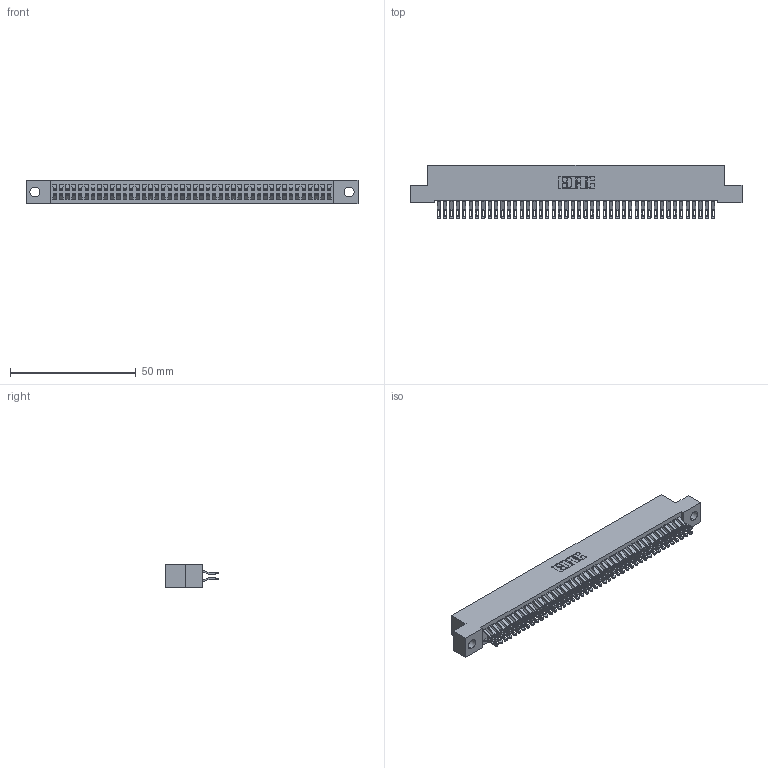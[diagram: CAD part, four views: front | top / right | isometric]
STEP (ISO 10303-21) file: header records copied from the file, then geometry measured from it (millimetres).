
FILE_DESCRIPTION (( 'STEP AP203' ), '1' );
FILE_NAME ('392-088-555-204.STEP', '2018-08-18T06:23:20', ( '' ), ( '' ), 'SwSTEP 2.0', 'SolidWorks 2016', '' );
FILE_SCHEMA (( 'CONFIG_CONTROL_DESIGN' ));
Length unit declared in the file: inch
Products named in the file (3): 345-292-001_555 Tail; 392-088-555-204; 342 Part_.156 TH
Assembly tree (89 placements, depth 2):
  392-088-555-204
    342 Part_.156 TH
    345-292-001_555 Tail  x88
Bounding box: 132.08 x 21.47 x 9.4 mm (x, y, z)
Volume: 12034.4 mm3; surface area: 20313.9 mm2
Topology: 89 solids, 89 shells, 5214 faces, 16403 edges, 10934 vertices
Faces by surface type: plane 3058, cylinder 2156
Entity records: 28245 total; most frequent: CARTESIAN_POINT 4712, ORIENTED_EDGE 4618, DIRECTION 3993, EDGE_CURVE 2309, VECTOR 2161, LINE 2161, VERTEX_POINT 1538, AXIS2_PLACEMENT_3D 916
